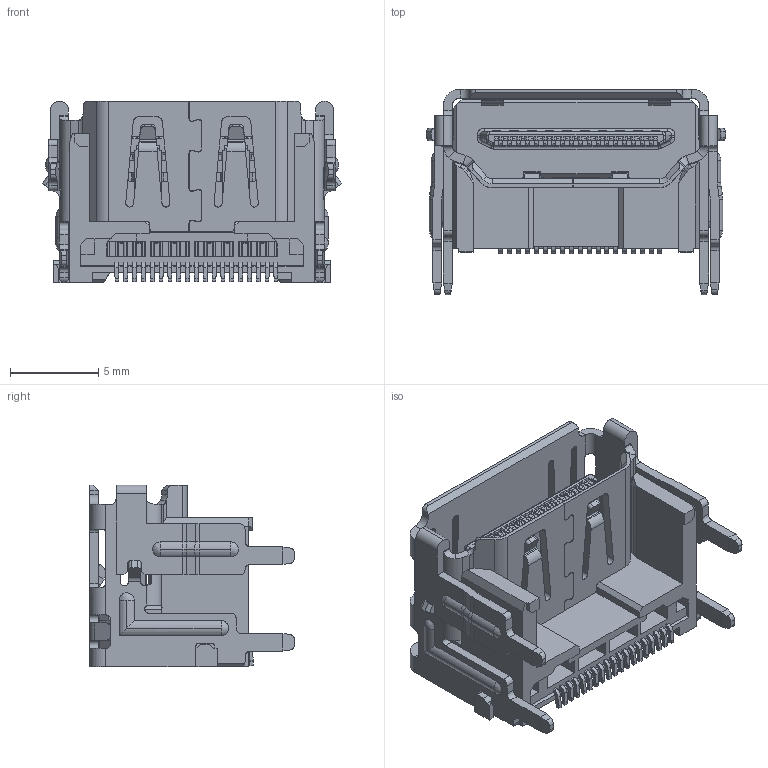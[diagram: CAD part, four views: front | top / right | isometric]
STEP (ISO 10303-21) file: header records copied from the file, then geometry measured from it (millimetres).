
FILE_DESCRIPTION (( 'STEP AP214' ), '1' );
FILE_NAME ('694D119-165-211.STEP', '2021-01-13T17:25:38', ( '' ), ( '' ), 'SwSTEP 2.0', 'SolidWorks 2020', '' );
FILE_SCHEMA (( 'AUTOMOTIVE_DESIGN' ));
Length unit declared in the file: millimetre
Products named in the file (3): Shell 694D119-X65-211; Insulator 694D119-X65-211; 694D119-165-211
Assembly tree (2 placements, depth 2):
  694D119-165-211
    Insulator 694D119-X65-211
    Shell 694D119-X65-211
Bounding box: 16.93 x 11.6 x 10.3 mm (x, y, z)
Volume: 494 mm3; surface area: 1799.9 mm2
Topology: 2 solids, 2 shells, 2616 faces, 7283 edges, 4606 vertices
Faces by surface type: plane 1649, cylinder 776, bspline 102, sphere 78, cone 11
Entity records: 95537 total; most frequent: CARTESIAN_POINT 25654, ORIENTED_EDGE 14458, DIRECTION 10791, EDGE_CURVE 7229, VERTEX_POINT 4606, LINE 4227, VECTOR 4227, AXIS2_PLACEMENT_3D 3282
